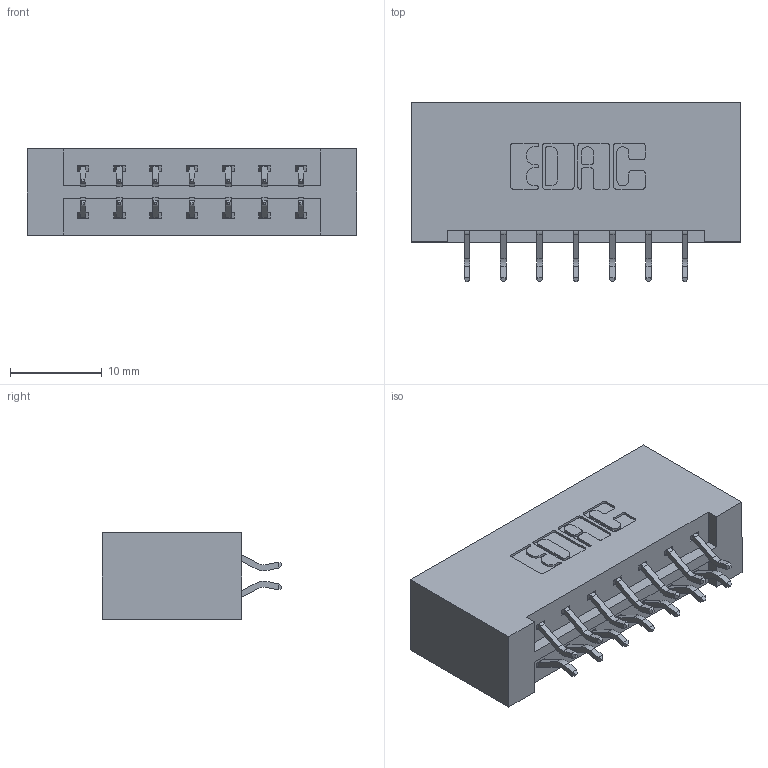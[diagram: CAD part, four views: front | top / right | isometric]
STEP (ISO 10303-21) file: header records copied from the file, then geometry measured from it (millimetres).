
FILE_DESCRIPTION (( 'STEP AP203' ), '1' );
FILE_NAME ('333-014-556-201.STEP', '2018-08-01T02:58:25', ( '' ), ( '' ), 'SwSTEP 2.0', 'SolidWorks 2016', '' );
FILE_SCHEMA (( 'CONFIG_CONTROL_DESIGN' ));
Length unit declared in the file: inch
Products named in the file (3): 333-014-556-201; 345-292-001_556 Tail; 333 Part_Lugless
Assembly tree (15 placements, depth 2):
  333-014-556-201
    333 Part_Lugless
    345-292-001_556 Tail  x14
Bounding box: 35.99 x 19.57 x 9.4 mm (x, y, z)
Volume: 3978.9 mm3; surface area: 4338.5 mm2
Topology: 15 solids, 15 shells, 918 faces, 2709 edges, 1786 vertices
Faces by surface type: plane 626, cylinder 292
Entity records: 8973 total; most frequent: CARTESIAN_POINT 1542, ORIENTED_EDGE 1466, DIRECTION 1361, EDGE_CURVE 733, LINE 605, VECTOR 605, VERTEX_POINT 486, AXIS2_PLACEMENT_3D 378
